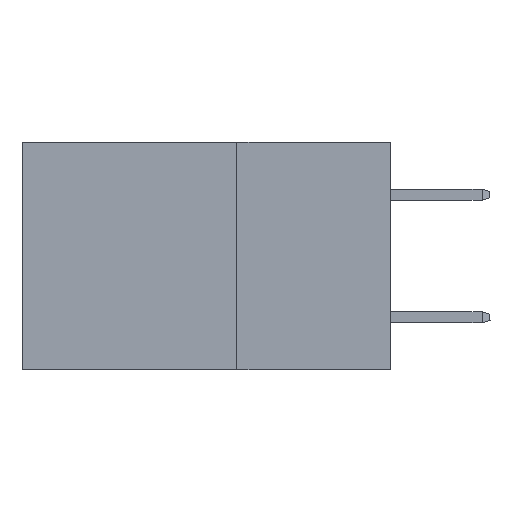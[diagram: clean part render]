
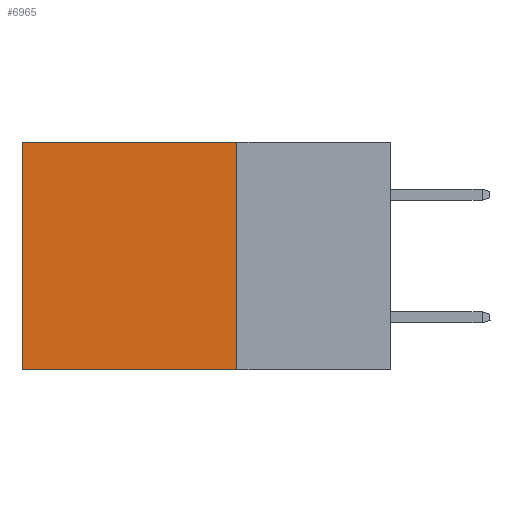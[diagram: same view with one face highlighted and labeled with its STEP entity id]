
A CAD part, left-side view. The second image highlights one B-rep face of the part: STEP entity #6965.
In plain terms, the highlighted planar face has unit normal (-1, 0, 0).
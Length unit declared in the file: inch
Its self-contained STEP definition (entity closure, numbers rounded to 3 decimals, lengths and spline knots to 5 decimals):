
#516 = LINE ( 'NONE', #1099, #6404 ) ;
#640 = ORIENTED_EDGE ( 'NONE', *, *, #1612, .T. ) ;
#925 = ORIENTED_EDGE ( 'NONE', *, *, #7165, .F. ) ;
#1003 = ORIENTED_EDGE ( 'NONE', *, *, #12987, .T. ) ;
#1099 = CARTESIAN_POINT ( 'NONE',  ( 0.2875, 0.25, -0.37 ) ) ;
#1612 = EDGE_CURVE ( 'NONE', #4780, #2931, #16494, .T. ) ;
#2472 = DIRECTION ( 'NONE',  ( 0., 0., -1. ) ) ;
#2693 = LINE ( 'NONE', #3753, #8631 ) ;
#2716 = CARTESIAN_POINT ( 'NONE',  ( 0.2875, 0.25, 0. ) ) ;
#2743 = DIRECTION ( 'NONE',  ( 0., 0., -1. ) ) ;
#2931 = VERTEX_POINT ( 'NONE', #5020 ) ;
#3753 = CARTESIAN_POINT ( 'NONE',  ( 0.2875, 0.6, 0. ) ) ;
#4494 = DIRECTION ( 'NONE',  ( 0., 1., 0. ) ) ;
#4780 = VERTEX_POINT ( 'NONE', #2716 ) ;
#5020 = CARTESIAN_POINT ( 'NONE',  ( 0.2875, 0.6, 0. ) ) ;
#5853 = CARTESIAN_POINT ( 'NONE',  ( 0.2875, 0.25, 0. ) ) ;
#6404 = VECTOR ( 'NONE', #10828, 39.37008 ) ;
#6659 = CARTESIAN_POINT ( 'NONE',  ( 0.2875, 0.25, -0.37 ) ) ;
#6965 = ADVANCED_FACE ( 'NONE', ( #15275 ), #17961, .F. ) ;
#7165 = EDGE_CURVE ( 'NONE', #4780, #9392, #11779, .T. ) ;
#8067 = CARTESIAN_POINT ( 'NONE',  ( 0.2875, 0.25, 0. ) ) ;
#8631 = VECTOR ( 'NONE', #13566, 39.37008 ) ;
#9064 = CARTESIAN_POINT ( 'NONE',  ( 0.2875, 0.6, -0.37 ) ) ;
#9392 = VERTEX_POINT ( 'NONE', #6659 ) ;
#9494 = AXIS2_PLACEMENT_3D ( 'NONE', #8067, #10811, #2472 ) ;
#9652 = VECTOR ( 'NONE', #2743, 39.37008 ) ;
#9698 = CARTESIAN_POINT ( 'NONE',  ( 0.2875, 0.25, 0. ) ) ;
#10811 = DIRECTION ( 'NONE',  ( 1., 0., 0. ) ) ;
#10828 = DIRECTION ( 'NONE',  ( 0., 1., 0. ) ) ;
#11779 = LINE ( 'NONE', #9698, #9652 ) ;
#12344 = VECTOR ( 'NONE', #4494, 39.37008 ) ;
#12506 = EDGE_LOOP ( 'NONE', ( #1003, #16225, #925, #640 ) ) ;
#12987 = EDGE_CURVE ( 'NONE', #2931, #15770, #2693, .T. ) ;
#13566 = DIRECTION ( 'NONE',  ( 0., 0., -1. ) ) ;
#14206 = EDGE_CURVE ( 'NONE', #9392, #15770, #516, .T. ) ;
#15275 = FACE_OUTER_BOUND ( 'NONE', #12506, .T. ) ;
#15770 = VERTEX_POINT ( 'NONE', #9064 ) ;
#16225 = ORIENTED_EDGE ( 'NONE', *, *, #14206, .F. ) ;
#16494 = LINE ( 'NONE', #5853, #12344 ) ;
#17961 = PLANE ( 'NONE',  #9494 ) ;
